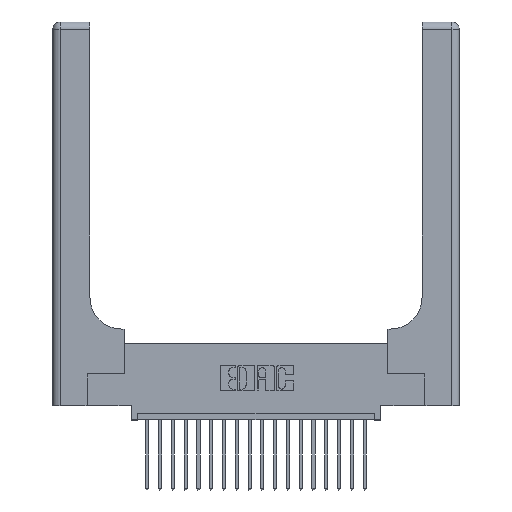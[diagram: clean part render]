
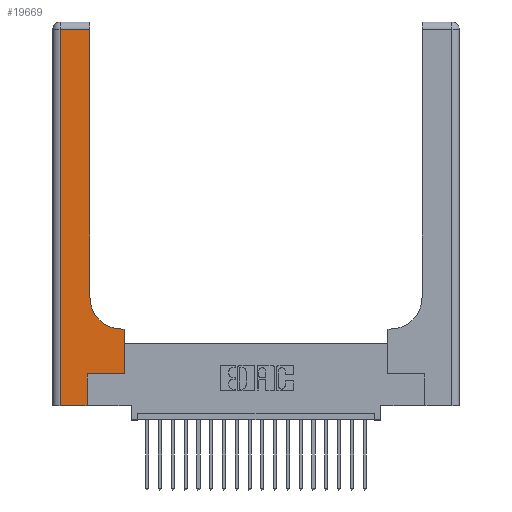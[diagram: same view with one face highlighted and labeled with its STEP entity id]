
A CAD part, top view. The second image highlights one B-rep face of the part: STEP entity #19669.
In plain terms, the highlighted planar face has unit normal (0, 0, 1).
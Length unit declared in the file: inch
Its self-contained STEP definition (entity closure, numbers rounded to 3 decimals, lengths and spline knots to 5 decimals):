
#57 = EDGE_CURVE ( 'NONE', #14559, #3593, #19109, .T. ) ;
#180 = DIRECTION ( 'NONE',  ( 1., 0., 0. ) ) ;
#227 = ORIENTED_EDGE ( 'NONE', *, *, #11402, .T. ) ;
#355 = DIRECTION ( 'NONE',  ( 1., 0., 0. ) ) ;
#975 = VERTEX_POINT ( 'NONE', #12591 ) ;
#1787 = DIRECTION ( 'NONE',  ( 0., 1., 0. ) ) ;
#2096 = VECTOR ( 'NONE', #7574, 39.37008 ) ;
#2246 = DIRECTION ( 'NONE',  ( 0., 1., 0. ) ) ;
#2644 = LINE ( 'NONE', #14922, #15660 ) ;
#3143 = VERTEX_POINT ( 'NONE', #13740 ) ;
#3263 = EDGE_CURVE ( 'NONE', #3593, #3143, #20869, .T. ) ;
#3593 = VERTEX_POINT ( 'NONE', #10655 ) ;
#3613 = CARTESIAN_POINT ( 'NONE',  ( 0.269, 0., 0.37 ) ) ;
#4115 = VERTEX_POINT ( 'NONE', #6574 ) ;
#4178 = VERTEX_POINT ( 'NONE', #5006 ) ;
#4935 = DIRECTION ( 'NONE',  ( -1., 0., 0. ) ) ;
#5006 = CARTESIAN_POINT ( 'NONE',  ( 0.06, 0., 0.37 ) ) ;
#5723 = CARTESIAN_POINT ( 'NONE',  ( 0.269, 0.25, 0.37 ) ) ;
#5769 = ORIENTED_EDGE ( 'NONE', *, *, #57, .T. ) ;
#5858 = VERTEX_POINT ( 'NONE', #16595 ) ;
#5938 = VERTEX_POINT ( 'NONE', #12317 ) ;
#6174 = DIRECTION ( 'NONE',  ( -1., 0., 0. ) ) ;
#6574 = CARTESIAN_POINT ( 'NONE',  ( 0.269, 0., 0.37 ) ) ;
#6698 = VECTOR ( 'NONE', #355, 39.37008 ) ;
#6771 = CARTESIAN_POINT ( 'NONE',  ( 0.5585, 0.25, 0.37 ) ) ;
#7335 = EDGE_CURVE ( 'NONE', #4115, #5938, #11284, .T. ) ;
#7487 = LINE ( 'NONE', #15248, #16004 ) ;
#7574 = DIRECTION ( 'NONE',  ( 0., -1., 0. ) ) ;
#8095 = EDGE_CURVE ( 'NONE', #975, #14559, #7487, .T. ) ;
#8640 = ORIENTED_EDGE ( 'NONE', *, *, #9713, .T. ) ;
#9023 = LINE ( 'NONE', #12693, #2096 ) ;
#9645 = CARTESIAN_POINT ( 'NONE',  ( 0., 0., 0.37 ) ) ;
#9713 = EDGE_CURVE ( 'NONE', #4178, #4115, #13542, .T. ) ;
#9933 = EDGE_CURVE ( 'NONE', #3143, #5858, #2644, .T. ) ;
#10326 = DIRECTION ( 'NONE',  ( 0., 0., -1. ) ) ;
#10655 = CARTESIAN_POINT ( 'NONE',  ( 0.2915, 0.85, 0.37 ) ) ;
#10894 = ORIENTED_EDGE ( 'NONE', *, *, #3263, .T. ) ;
#10979 = AXIS2_PLACEMENT_3D ( 'NONE', #12624, #15993, #17878 ) ;
#11284 = LINE ( 'NONE', #3613, #13401 ) ;
#11402 = EDGE_CURVE ( 'NONE', #5938, #19939, #20836, .T. ) ;
#11561 = AXIS2_PLACEMENT_3D ( 'NONE', #13578, #10326, #180 ) ;
#11719 = FACE_OUTER_BOUND ( 'NONE', #18837, .T. ) ;
#12317 = CARTESIAN_POINT ( 'NONE',  ( 0.269, 0.25, 0.37 ) ) ;
#12497 = ORIENTED_EDGE ( 'NONE', *, *, #7335, .T. ) ;
#12591 = CARTESIAN_POINT ( 'NONE',  ( 0.5585, 0.6, 0.37 ) ) ;
#12624 = CARTESIAN_POINT ( 'NONE',  ( 0., 3., 0.37 ) ) ;
#12693 = CARTESIAN_POINT ( 'NONE',  ( 0.06, 3., 0.37 ) ) ;
#12820 = CARTESIAN_POINT ( 'NONE',  ( 0.5415, 0.6, 0.37 ) ) ;
#13401 = VECTOR ( 'NONE', #1787, 39.37008 ) ;
#13542 = LINE ( 'NONE', #9645, #16449 ) ;
#13578 = CARTESIAN_POINT ( 'NONE',  ( 0.5415, 0.85, 0.37 ) ) ;
#13725 = VECTOR ( 'NONE', #16962, 39.37008 ) ;
#13740 = CARTESIAN_POINT ( 'NONE',  ( 0.2915, 2.94, 0.37 ) ) ;
#14105 = EDGE_CURVE ( 'NONE', #19939, #975, #16105, .T. ) ;
#14485 = ORIENTED_EDGE ( 'NONE', *, *, #14105, .T. ) ;
#14559 = VERTEX_POINT ( 'NONE', #12820 ) ;
#14922 = CARTESIAN_POINT ( 'NONE',  ( 0., 2.94, 0.37 ) ) ;
#15248 = CARTESIAN_POINT ( 'NONE',  ( 0.2915, 0.6, 0.37 ) ) ;
#15484 = VECTOR ( 'NONE', #2246, 39.37008 ) ;
#15660 = VECTOR ( 'NONE', #6174, 39.37008 ) ;
#15669 = ORIENTED_EDGE ( 'NONE', *, *, #9933, .T. ) ;
#15993 = DIRECTION ( 'NONE',  ( 0., 0., -1. ) ) ;
#16004 = VECTOR ( 'NONE', #4935, 39.37008 ) ;
#16105 = LINE ( 'NONE', #17132, #13725 ) ;
#16449 = VECTOR ( 'NONE', #21572, 39.37008 ) ;
#16595 = CARTESIAN_POINT ( 'NONE',  ( 0.06, 2.94, 0.37 ) ) ;
#16962 = DIRECTION ( 'NONE',  ( 0., 1., 0. ) ) ;
#17132 = CARTESIAN_POINT ( 'NONE',  ( 0.5585, 0.25, 0.37 ) ) ;
#17488 = PLANE ( 'NONE',  #10979 ) ;
#17878 = DIRECTION ( 'NONE',  ( -1., 0., 0. ) ) ;
#18837 = EDGE_LOOP ( 'NONE', ( #10894, #15669, #20529, #8640, #12497, #227, #14485, #21250, #5769 ) ) ;
#19109 = CIRCLE ( 'NONE', #11561, 0.25 ) ;
#19138 = CARTESIAN_POINT ( 'NONE',  ( 0.2915, 3., 0.37 ) ) ;
#19669 = ADVANCED_FACE ( 'NONE', ( #11719 ), #17488, .F. ) ;
#19712 = EDGE_CURVE ( 'NONE', #5858, #4178, #9023, .T. ) ;
#19939 = VERTEX_POINT ( 'NONE', #6771 ) ;
#20529 = ORIENTED_EDGE ( 'NONE', *, *, #19712, .T. ) ;
#20836 = LINE ( 'NONE', #5723, #6698 ) ;
#20869 = LINE ( 'NONE', #19138, #15484 ) ;
#21250 = ORIENTED_EDGE ( 'NONE', *, *, #8095, .T. ) ;
#21572 = DIRECTION ( 'NONE',  ( 1., 0., 0. ) ) ;
